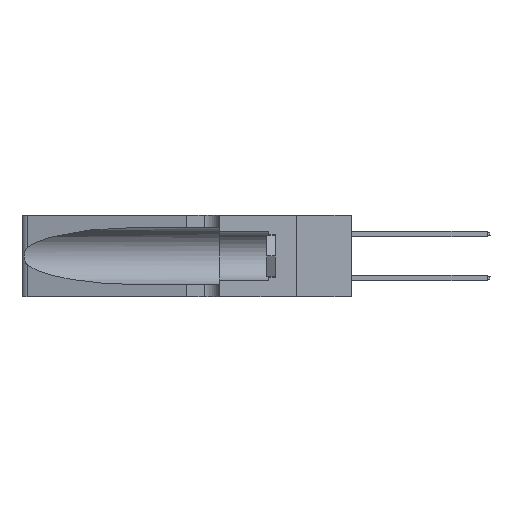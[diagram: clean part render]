
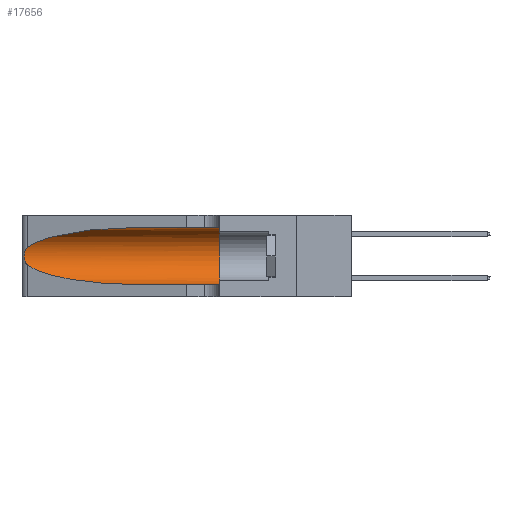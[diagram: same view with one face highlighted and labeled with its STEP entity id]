
A CAD part, left-side view. The second image highlights one B-rep face of the part: STEP entity #17656.
In plain terms, the highlighted cylindrical face has radius 3.308 mm (diameter 6.617 mm), a partial arc.
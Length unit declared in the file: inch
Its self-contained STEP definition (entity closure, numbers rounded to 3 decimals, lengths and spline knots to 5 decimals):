
#1179 = CARTESIAN_POINT ( 'NONE',  ( 0.25639, 1.23186, 0.15144 ) ) ;
#1937 = CARTESIAN_POINT ( 'NONE',  ( 0.1305, 0.35, 0.185 ) ) ;
#2228 = DIRECTION ( 'NONE',  ( 0., -1., 0. ) ) ;
#3075 = EDGE_CURVE ( 'NONE', #17795, #33962, #29889, .T. ) ;
#3319 = LINE ( 'NONE', #17671, #29832 ) ;
#3716 = VECTOR ( 'NONE', #10716, 39.37008 ) ;
#4128 = ORIENTED_EDGE ( 'NONE', *, *, #4861, .T. ) ;
#4244 = CARTESIAN_POINT ( 'NONE',  ( 0.26017, 1.23833, 0.17102 ) ) ;
#4347 = DIRECTION ( 'NONE',  ( 0., -1., 0. ) ) ;
#4861 = EDGE_CURVE ( 'NONE', #34951, #28721, #8631, .T. ) ;
#4922 = CYLINDRICAL_SURFACE ( 'NONE', #18165, 0.13025 ) ;
#6233 = CARTESIAN_POINT ( 'NONE',  ( 0.1305, 0.72297, 0.31525 ) ) ;
#7580 = CARTESIAN_POINT ( 'NONE',  ( 0.25856, 1.23593, 0.16098 ) ) ;
#8108 = EDGE_CURVE ( 'NONE', #28721, #27186, #41334, .T. ) ;
#8631 = B_SPLINE_CURVE_WITH_KNOTS ( 'NONE', 3,
 ( #30957, #37314, #40944, #31239, #14231, #21064, #30671, #10930, #4244, #7580, #33982, #1179, #37749, #17428 ),
 .UNSPECIFIED., .F., .F.,
 ( 4, 2, 2, 2, 2, 2, 4 ),
 ( 0., 0.00027, 0.00053, 0.00107, 0.0016, 0.00187, 0.00214 ),
 .UNSPECIFIED. ) ;
#8734 = CARTESIAN_POINT ( 'NONE',  ( 0.1305, 0.72297, 0.31525 ) ) ;
#9445 = EDGE_CURVE ( 'NONE', #30476, #34951, #36273, .T. ) ;
#9857 = EDGE_CURVE ( 'NONE', #27186, #33962, #3319, .T. ) ;
#9996 = CARTESIAN_POINT ( 'NONE',  ( 0.1305, 0.72297, 0.05475 ) ) ;
#10716 = DIRECTION ( 'NONE',  ( 0., -1., 0. ) ) ;
#10930 = CARTESIAN_POINT ( 'NONE',  ( 0.26075, 1.23896, 0.178 ) ) ;
#11346 = ORIENTED_EDGE ( 'NONE', *, *, #8108, .T. ) ;
#11667 = FACE_OUTER_BOUND ( 'NONE', #16587, .T. ) ;
#11980 = CARTESIAN_POINT ( 'NONE',  ( 0.1305, 1.61858, 0.185 ) ) ;
#14231 = CARTESIAN_POINT ( 'NONE',  ( 0.25854, 1.2359, 0.20912 ) ) ;
#15083 = CARTESIAN_POINT ( 'NONE',  ( 0.25487, 1.22718, 0.22369 ) ) ;
#16587 = EDGE_LOOP ( 'NONE', ( #21234, #4128, #11346, #29666, #28395, #40146 ) ) ;
#17428 = CARTESIAN_POINT ( 'NONE',  ( 0.25487, 1.22718, 0.14631 ) ) ;
#17656 = ADVANCED_FACE ( 'NONE', ( #11667 ), #4922, .F. ) ;
#17671 = CARTESIAN_POINT ( 'NONE',  ( 0.1305, 1.61858, 0.05475 ) ) ;
#17795 = VERTEX_POINT ( 'NONE', #33159 ) ;
#18165 = AXIS2_PLACEMENT_3D ( 'NONE', #11980, #2228, #34912 ) ;
#19135 = EDGE_CURVE ( 'NONE', #30476, #17795, #38497, .T. ) ;
#21064 = CARTESIAN_POINT ( 'NONE',  ( 0.26018, 1.23835, 0.19895 ) ) ;
#21234 = ORIENTED_EDGE ( 'NONE', *, *, #9445, .T. ) ;
#23463 = CARTESIAN_POINT ( 'NONE',  ( 0.1305, 0.35, 0.05475 ) ) ;
#25656 = CARTESIAN_POINT ( 'NONE',  ( 0.18966, 0.96281, 0.05475 ) ) ;
#27186 = VERTEX_POINT ( 'NONE', #9996 ) ;
#27582 = AXIS2_PLACEMENT_3D ( 'NONE', #1937, #34606, #37939 ) ;
#28395 = ORIENTED_EDGE ( 'NONE', *, *, #3075, .F. ) ;
#28721 = VERTEX_POINT ( 'NONE', #38010 ) ;
#28755 = CARTESIAN_POINT ( 'NONE',  ( 0.18966, 0.96281, 0.31525 ) ) ;
#29666 = ORIENTED_EDGE ( 'NONE', *, *, #9857, .T. ) ;
#29832 = VECTOR ( 'NONE', #4347, 39.37008 ) ;
#29889 = CIRCLE ( 'NONE', #27582, 0.13025 ) ;
#30476 = VERTEX_POINT ( 'NONE', #6233 ) ;
#30671 = CARTESIAN_POINT ( 'NONE',  ( 0.26075, 1.23896, 0.19203 ) ) ;
#30957 = CARTESIAN_POINT ( 'NONE',  ( 0.25487, 1.22718, 0.22369 ) ) ;
#31239 = CARTESIAN_POINT ( 'NONE',  ( 0.25787, 1.23484, 0.2124 ) ) ;
#32187 = CARTESIAN_POINT ( 'NONE',  ( 0.25487, 1.22718, 0.14631 ) ) ;
#32324 = CARTESIAN_POINT ( 'NONE',  ( 0.1305, 0.72297, 0.05475 ) ) ;
#33159 = CARTESIAN_POINT ( 'NONE',  ( 0.1305, 0.35, 0.31525 ) ) ;
#33774 = CARTESIAN_POINT ( 'NONE',  ( 0.1305, 1.61858, 0.31525 ) ) ;
#33962 = VERTEX_POINT ( 'NONE', #23463 ) ;
#33982 = CARTESIAN_POINT ( 'NONE',  ( 0.25789, 1.23486, 0.15765 ) ) ;
#34606 = DIRECTION ( 'NONE',  ( 0., 1., 0. ) ) ;
#34912 = DIRECTION ( 'NONE',  ( 0., 0., -1. ) ) ;
#34951 = VERTEX_POINT ( 'NONE', #41516 ) ;
#34984 = CARTESIAN_POINT ( 'NONE',  ( 0.2373, 1.15595, 0.28018 ) ) ;
#36273 =( BOUNDED_CURVE ( )  B_SPLINE_CURVE ( 3, ( #8734, #28755, #34984, #15083 ),
 .UNSPECIFIED., .F., .F. ) 
 B_SPLINE_CURVE_WITH_KNOTS ( ( 4, 4 ),
 ( 1.5708, 2.84003 ),
 .UNSPECIFIED. ) 
 CURVE ( )  GEOMETRIC_REPRESENTATION_ITEM ( )  RATIONAL_B_SPLINE_CURVE ( ( 1., 0.87, 0.87, 1. ) ) 
 REPRESENTATION_ITEM ( '' )  );
#37314 = CARTESIAN_POINT ( 'NONE',  ( 0.25555, 1.22994, 0.2215 ) ) ;
#37749 = CARTESIAN_POINT ( 'NONE',  ( 0.25555, 1.22993, 0.14849 ) ) ;
#37939 = DIRECTION ( 'NONE',  ( 0., 0., 1. ) ) ;
#38010 = CARTESIAN_POINT ( 'NONE',  ( 0.25487, 1.22718, 0.14631 ) ) ;
#38409 = CARTESIAN_POINT ( 'NONE',  ( 0.2373, 1.15595, 0.08982 ) ) ;
#38497 = LINE ( 'NONE', #33774, #3716 ) ;
#40146 = ORIENTED_EDGE ( 'NONE', *, *, #19135, .F. ) ;
#40944 = CARTESIAN_POINT ( 'NONE',  ( 0.25639, 1.23184, 0.21858 ) ) ;
#41334 =( BOUNDED_CURVE ( )  B_SPLINE_CURVE ( 3, ( #32187, #38409, #25656, #32324 ),
 .UNSPECIFIED., .F., .F. ) 
 B_SPLINE_CURVE_WITH_KNOTS ( ( 4, 4 ),
 ( 3.44316, 4.71239 ),
 .UNSPECIFIED. ) 
 CURVE ( )  GEOMETRIC_REPRESENTATION_ITEM ( )  RATIONAL_B_SPLINE_CURVE ( ( 1., 0.87, 0.87, 1. ) ) 
 REPRESENTATION_ITEM ( '' )  );
#41516 = CARTESIAN_POINT ( 'NONE',  ( 0.25487, 1.22718, 0.22369 ) ) ;
